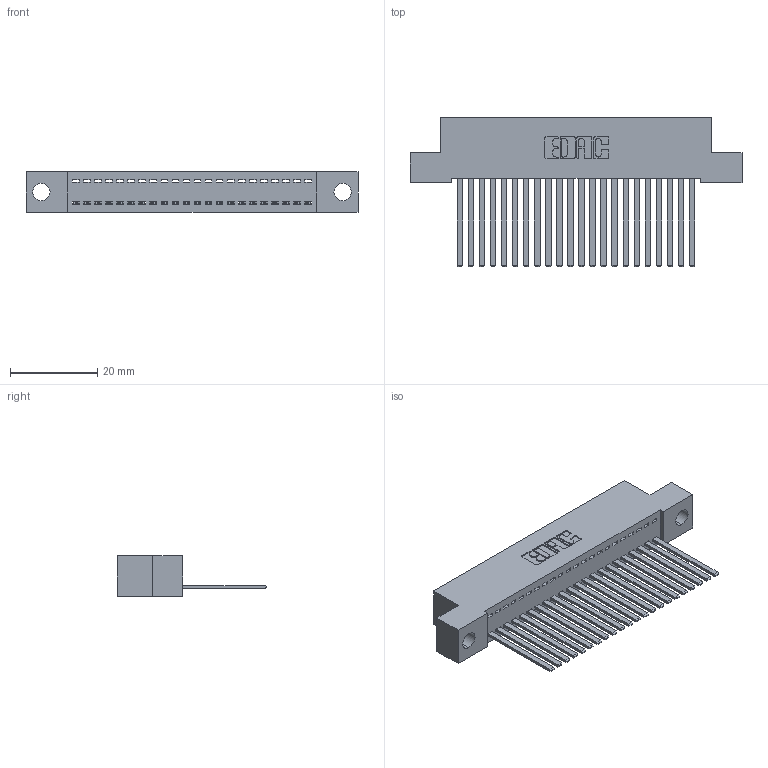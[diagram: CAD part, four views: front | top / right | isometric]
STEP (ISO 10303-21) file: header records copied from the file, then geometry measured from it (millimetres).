
FILE_DESCRIPTION (( 'STEP AP203' ), '1' );
FILE_NAME ('392-022-544-104.STEP', '2019-10-07T06:24:57', ( '' ), ( '' ), 'SwSTEP 2.0', 'SolidWorks 2016', '' );
FILE_SCHEMA (( 'CONFIG_CONTROL_DESIGN' ));
Length unit declared in the file: inch
Products named in the file (3): 342 Part_.156 TH; 345-292-001_345-293-144; 392-022-544-104
Assembly tree (23 placements, depth 2):
  392-022-544-104
    342 Part_.156 TH
    345-292-001_345-293-144  x22
Bounding box: 76.2 x 34.3 x 9.4 mm (x, y, z)
Volume: 6775.3 mm3; surface area: 10119.7 mm2
Topology: 23 solids, 23 shells, 1254 faces, 3775 edges, 2486 vertices
Faces by surface type: plane 902, cylinder 352
Entity records: 15723 total; most frequent: CARTESIAN_POINT 2720, ORIENTED_EDGE 2678, DIRECTION 2331, EDGE_CURVE 1339, VECTOR 1215, LINE 1215, VERTEX_POINT 890, AXIS2_PLACEMENT_3D 558
